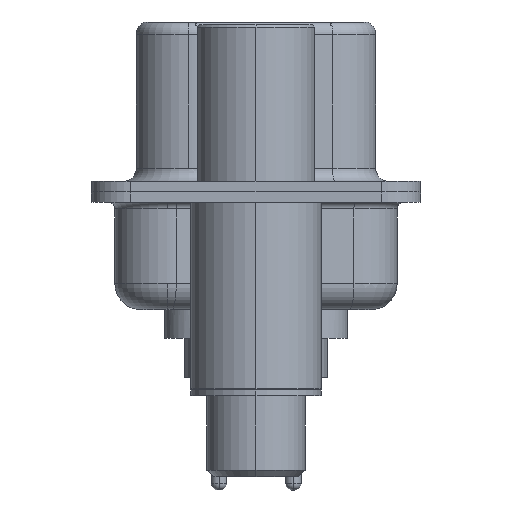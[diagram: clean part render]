
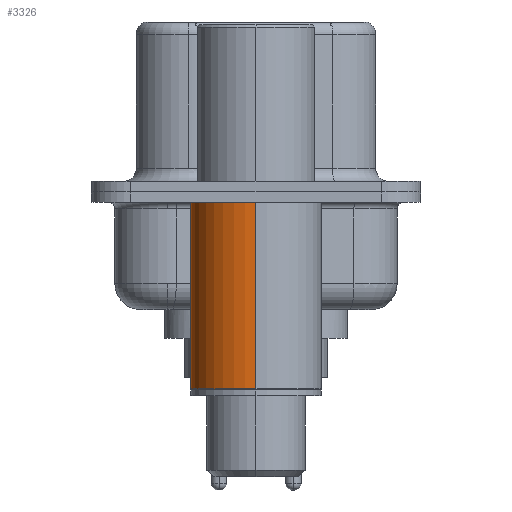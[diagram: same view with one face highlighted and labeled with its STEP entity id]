
A CAD part, left-side view. The second image highlights one B-rep face of the part: STEP entity #3326.
In plain terms, the highlighted cylindrical face has radius 2.5 mm (diameter 5 mm), a partial arc.
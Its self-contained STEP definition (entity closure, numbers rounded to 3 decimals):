
#5 = AXIS2_PLACEMENT_3D ( 'NONE', #21594, #10096, #10109 ) ;
#55 = LINE ( 'NONE', #17078, #14475 ) ;
#578 = EDGE_CURVE ( 'NONE', #1710, #10261, #12830, .T. ) ;
#604 = EDGE_CURVE ( 'NONE', #22247, #10261, #12268, .T. ) ;
#1710 = VERTEX_POINT ( 'NONE', #6045 ) ;
#3326 = ADVANCED_FACE ( 'NONE', ( #18595 ), #8428, .T. ) ;
#4417 = DIRECTION ( 'NONE',  ( 1., 0., 0. ) ) ;
#4591 = DIRECTION ( 'NONE',  ( 0., 0., 1. ) ) ;
#4728 = EDGE_CURVE ( 'NONE', #5967, #1710, #21916, .T. ) ;
#4734 = CARTESIAN_POINT ( 'NONE',  ( -2.5, 0., -0.4 ) ) ;
#4905 = CARTESIAN_POINT ( 'NONE',  ( 0., 0., -0.4 ) ) ;
#5334 = ORIENTED_EDGE ( 'NONE', *, *, #4728, .T. ) ;
#5967 = VERTEX_POINT ( 'NONE', #7097 ) ;
#6045 = CARTESIAN_POINT ( 'NONE',  ( -2.5, 0., -7.525 ) ) ;
#6229 = DIRECTION ( 'NONE',  ( 0., 0., 1. ) ) ;
#7097 = CARTESIAN_POINT ( 'NONE',  ( 2.5, 0., -7.525 ) ) ;
#7574 = ORIENTED_EDGE ( 'NONE', *, *, #604, .F. ) ;
#8155 = DIRECTION ( 'NONE',  ( 0., 0., 1. ) ) ;
#8428 = CYLINDRICAL_SURFACE ( 'NONE', #23270, 2.5 ) ;
#9522 = AXIS2_PLACEMENT_3D ( 'NONE', #4905, #4591, #4417 ) ;
#10096 = DIRECTION ( 'NONE',  ( 0., 0., 1. ) ) ;
#10109 = DIRECTION ( 'NONE',  ( 1., 0., 0. ) ) ;
#10219 = ORIENTED_EDGE ( 'NONE', *, *, #21150, .F. ) ;
#10261 = VERTEX_POINT ( 'NONE', #4734 ) ;
#11065 = DIRECTION ( 'NONE',  ( 1., 0., 0. ) ) ;
#11312 = CARTESIAN_POINT ( 'NONE',  ( -2.5, 0., 0.581 ) ) ;
#12268 = CIRCLE ( 'NONE', #9522, 2.5 ) ;
#12742 = CARTESIAN_POINT ( 'NONE',  ( 2.5, 0., -0.4 ) ) ;
#12830 = LINE ( 'NONE', #11312, #17102 ) ;
#14475 = VECTOR ( 'NONE', #6229, 1000. ) ;
#17078 = CARTESIAN_POINT ( 'NONE',  ( 2.5, 0., 0.581 ) ) ;
#17102 = VECTOR ( 'NONE', #8155, 1000. ) ;
#18595 = FACE_OUTER_BOUND ( 'NONE', #19342, .T. ) ;
#19342 = EDGE_LOOP ( 'NONE', ( #5334, #19575, #7574, #10219 ) ) ;
#19575 = ORIENTED_EDGE ( 'NONE', *, *, #578, .T. ) ;
#20820 = DIRECTION ( 'NONE',  ( 0., 0., 1. ) ) ;
#21150 = EDGE_CURVE ( 'NONE', #5967, #22247, #55, .T. ) ;
#21594 = CARTESIAN_POINT ( 'NONE',  ( 0., 0., -7.525 ) ) ;
#21916 = CIRCLE ( 'NONE', #5, 2.5 ) ;
#22247 = VERTEX_POINT ( 'NONE', #12742 ) ;
#22319 = CARTESIAN_POINT ( 'NONE',  ( 0., 0., 0.581 ) ) ;
#23270 = AXIS2_PLACEMENT_3D ( 'NONE', #22319, #20820, #11065 ) ;
